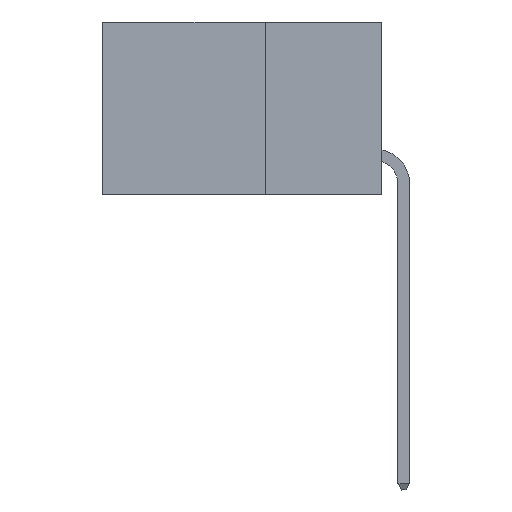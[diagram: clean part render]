
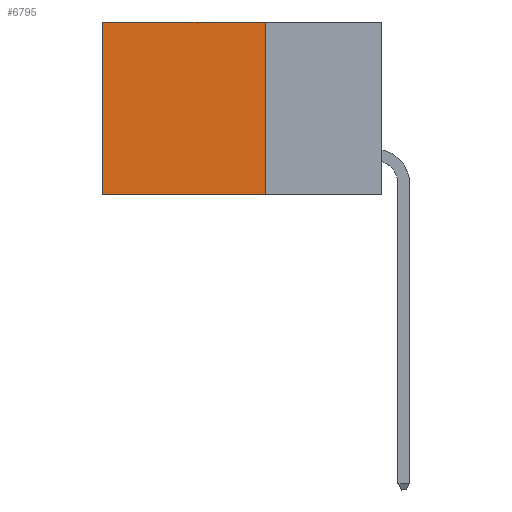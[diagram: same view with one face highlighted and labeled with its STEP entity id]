
A CAD part, left-side view. The second image highlights one B-rep face of the part: STEP entity #6795.
In plain terms, the highlighted planar face has unit normal (-1, 0, 0).
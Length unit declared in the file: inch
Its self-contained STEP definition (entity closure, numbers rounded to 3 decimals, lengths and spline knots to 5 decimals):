
#1105 = ORIENTED_EDGE ( 'NONE', *, *, #15683, .T. ) ;
#1879 = ORIENTED_EDGE ( 'NONE', *, *, #7301, .F. ) ;
#2136 = CARTESIAN_POINT ( 'NONE',  ( 0.2875, 0.6, -0.37 ) ) ;
#2410 = VERTEX_POINT ( 'NONE', #12221 ) ;
#4173 = DIRECTION ( 'NONE',  ( 0., 1., 0. ) ) ;
#4561 = VERTEX_POINT ( 'NONE', #2136 ) ;
#4729 = LINE ( 'NONE', #10186, #5774 ) ;
#5474 = DIRECTION ( 'NONE',  ( 0., 0., -1. ) ) ;
#5596 = EDGE_LOOP ( 'NONE', ( #1105, #9569, #1879, #6219 ) ) ;
#5682 = FACE_OUTER_BOUND ( 'NONE', #5596, .T. ) ;
#5774 = VECTOR ( 'NONE', #5474, 39.37008 ) ;
#6219 = ORIENTED_EDGE ( 'NONE', *, *, #9227, .T. ) ;
#6795 = ADVANCED_FACE ( 'NONE', ( #5682 ), #19704, .F. ) ;
#6885 = DIRECTION ( 'NONE',  ( 0., 0., -1. ) ) ;
#7301 = EDGE_CURVE ( 'NONE', #13767, #2410, #8719, .T. ) ;
#8271 = VERTEX_POINT ( 'NONE', #12878 ) ;
#8333 = DIRECTION ( 'NONE',  ( 1., 0., 0. ) ) ;
#8719 = LINE ( 'NONE', #18566, #18893 ) ;
#8808 = AXIS2_PLACEMENT_3D ( 'NONE', #13153, #8333, #11666 ) ;
#9227 = EDGE_CURVE ( 'NONE', #13767, #8271, #15716, .T. ) ;
#9569 = ORIENTED_EDGE ( 'NONE', *, *, #17361, .F. ) ;
#9647 = CARTESIAN_POINT ( 'NONE',  ( 0.2875, 0.25, 0. ) ) ;
#10186 = CARTESIAN_POINT ( 'NONE',  ( 0.2875, 0.6, 0. ) ) ;
#10754 = DIRECTION ( 'NONE',  ( 0., 1., 0. ) ) ;
#11666 = DIRECTION ( 'NONE',  ( 0., 0., -1. ) ) ;
#12221 = CARTESIAN_POINT ( 'NONE',  ( 0.2875, 0.25, -0.37 ) ) ;
#12878 = CARTESIAN_POINT ( 'NONE',  ( 0.2875, 0.6, 0. ) ) ;
#13153 = CARTESIAN_POINT ( 'NONE',  ( 0.2875, 0.25, 0. ) ) ;
#13175 = VECTOR ( 'NONE', #4173, 39.37008 ) ;
#13767 = VERTEX_POINT ( 'NONE', #9647 ) ;
#13796 = CARTESIAN_POINT ( 'NONE',  ( 0.2875, 0.25, -0.37 ) ) ;
#15106 = LINE ( 'NONE', #13796, #17408 ) ;
#15423 = CARTESIAN_POINT ( 'NONE',  ( 0.2875, 0.25, 0. ) ) ;
#15683 = EDGE_CURVE ( 'NONE', #8271, #4561, #4729, .T. ) ;
#15716 = LINE ( 'NONE', #15423, #13175 ) ;
#17361 = EDGE_CURVE ( 'NONE', #2410, #4561, #15106, .T. ) ;
#17408 = VECTOR ( 'NONE', #10754, 39.37008 ) ;
#18566 = CARTESIAN_POINT ( 'NONE',  ( 0.2875, 0.25, 0. ) ) ;
#18893 = VECTOR ( 'NONE', #6885, 39.37008 ) ;
#19704 = PLANE ( 'NONE',  #8808 ) ;
